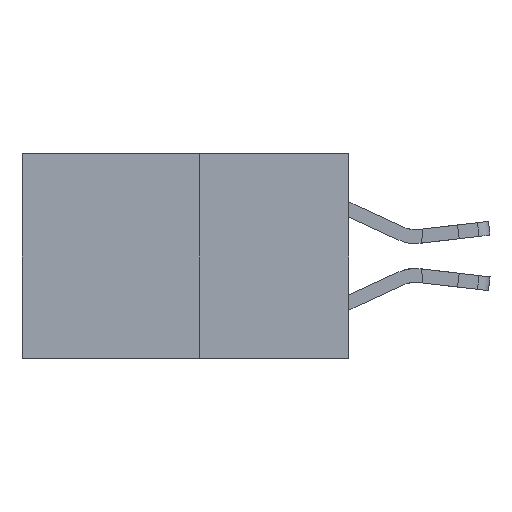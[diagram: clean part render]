
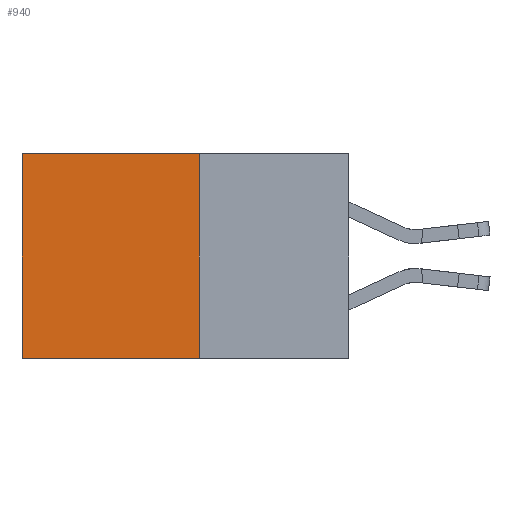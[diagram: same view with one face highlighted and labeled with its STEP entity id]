
A CAD part, left-side view. The second image highlights one B-rep face of the part: STEP entity #940.
In plain terms, the highlighted planar face has unit normal (-1, 0, 0).
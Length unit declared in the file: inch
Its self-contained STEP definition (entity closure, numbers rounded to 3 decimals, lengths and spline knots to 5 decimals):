
#940 = ADVANCED_FACE ( 'NONE', ( #18299 ), #10267, .F. ) ;
#1601 = VECTOR ( 'NONE', #7413, 39.37008 ) ;
#2839 = ORIENTED_EDGE ( 'NONE', *, *, #7640, .F. ) ;
#3941 = CARTESIAN_POINT ( 'NONE',  ( 0.277, 0.27, -0.37 ) ) ;
#4306 = EDGE_LOOP ( 'NONE', ( #5396, #2839, #18017, #11460 ) ) ;
#5152 = DIRECTION ( 'NONE',  ( 0., 1., 0. ) ) ;
#5153 = EDGE_CURVE ( 'NONE', #19122, #16022, #19271, .T. ) ;
#5396 = ORIENTED_EDGE ( 'NONE', *, *, #18687, .T. ) ;
#5886 = LINE ( 'NONE', #20222, #1601 ) ;
#6277 = CARTESIAN_POINT ( 'NONE',  ( 0.277, 0.59, -0.37 ) ) ;
#6352 = DIRECTION ( 'NONE',  ( 0., 0., -1. ) ) ;
#7378 = CARTESIAN_POINT ( 'NONE',  ( 0.277, 0.27, 0. ) ) ;
#7413 = DIRECTION ( 'NONE',  ( 0., 0., -1. ) ) ;
#7640 = EDGE_CURVE ( 'NONE', #18817, #21311, #18056, .T. ) ;
#8316 = VECTOR ( 'NONE', #5152, 39.37008 ) ;
#9271 = CARTESIAN_POINT ( 'NONE',  ( 0.277, 0.59, 0. ) ) ;
#10107 = CARTESIAN_POINT ( 'NONE',  ( 0.277, 0.27, -0.37 ) ) ;
#10267 = PLANE ( 'NONE',  #10847 ) ;
#10847 = AXIS2_PLACEMENT_3D ( 'NONE', #10107, #12712, #12454 ) ;
#11460 = ORIENTED_EDGE ( 'NONE', *, *, #5153, .T. ) ;
#11885 = VECTOR ( 'NONE', #6352, 39.37008 ) ;
#12454 = DIRECTION ( 'NONE',  ( 0., 0., -1. ) ) ;
#12712 = DIRECTION ( 'NONE',  ( 1., 0., 0. ) ) ;
#14066 = EDGE_CURVE ( 'NONE', #19122, #18817, #5886, .T. ) ;
#14387 = CARTESIAN_POINT ( 'NONE',  ( 0.277, 0.27, 0. ) ) ;
#14443 = VECTOR ( 'NONE', #16677, 39.37008 ) ;
#16022 = VERTEX_POINT ( 'NONE', #9271 ) ;
#16677 = DIRECTION ( 'NONE',  ( 0., 1., 0. ) ) ;
#18017 = ORIENTED_EDGE ( 'NONE', *, *, #14066, .F. ) ;
#18056 = LINE ( 'NONE', #3941, #8316 ) ;
#18299 = FACE_OUTER_BOUND ( 'NONE', #4306, .T. ) ;
#18687 = EDGE_CURVE ( 'NONE', #16022, #21311, #22121, .T. ) ;
#18817 = VERTEX_POINT ( 'NONE', #23001 ) ;
#19122 = VERTEX_POINT ( 'NONE', #7378 ) ;
#19271 = LINE ( 'NONE', #14387, #14443 ) ;
#20092 = CARTESIAN_POINT ( 'NONE',  ( 0.277, 0.59, -0.37 ) ) ;
#20222 = CARTESIAN_POINT ( 'NONE',  ( 0.277, 0.27, -0.37 ) ) ;
#21311 = VERTEX_POINT ( 'NONE', #20092 ) ;
#22121 = LINE ( 'NONE', #6277, #11885 ) ;
#23001 = CARTESIAN_POINT ( 'NONE',  ( 0.277, 0.27, -0.37 ) ) ;
